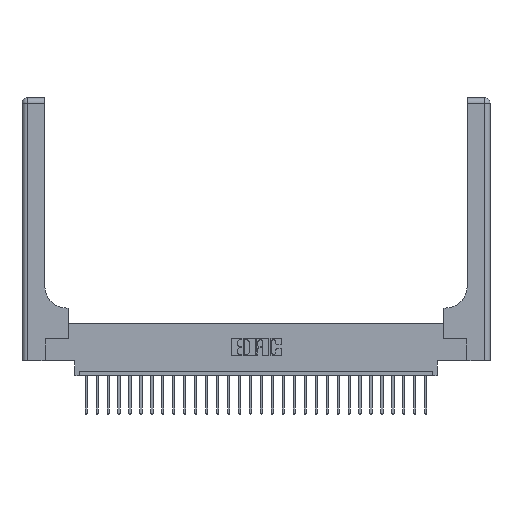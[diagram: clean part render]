
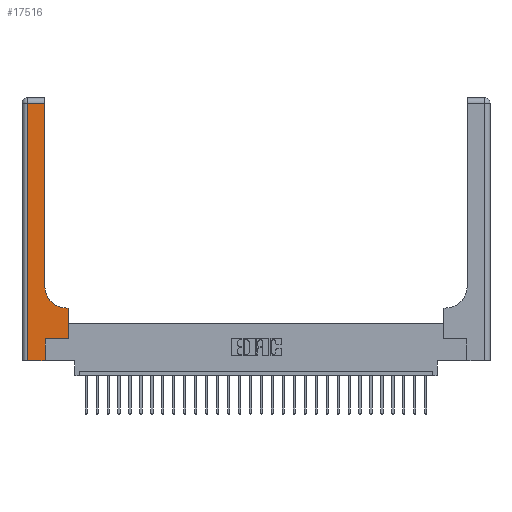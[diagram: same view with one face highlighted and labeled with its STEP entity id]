
A CAD part, top view. The second image highlights one B-rep face of the part: STEP entity #17516.
In plain terms, the highlighted planar face has unit normal (0, 0, 1).
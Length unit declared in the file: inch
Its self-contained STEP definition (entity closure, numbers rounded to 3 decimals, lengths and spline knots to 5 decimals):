
#828 = VERTEX_POINT ( 'NONE', #7912 ) ;
#926 = VECTOR ( 'NONE', #26371, 39.37008 ) ;
#1045 = LINE ( 'NONE', #6422, #16062 ) ;
#1408 = CARTESIAN_POINT ( 'NONE',  ( 0.26, 0.85, 0.37 ) ) ;
#1803 = LINE ( 'NONE', #7105, #24854 ) ;
#1862 = CARTESIAN_POINT ( 'NONE',  ( 0.51, 0.85, 0.37 ) ) ;
#2149 = ORIENTED_EDGE ( 'NONE', *, *, #23066, .T. ) ;
#2358 = LINE ( 'NONE', #22994, #5868 ) ;
#2744 = VECTOR ( 'NONE', #21874, 39.37008 ) ;
#4751 = EDGE_CURVE ( 'NONE', #7977, #6537, #1803, .T. ) ;
#5842 = CARTESIAN_POINT ( 'NONE',  ( 0.265, 0.25, 0.37 ) ) ;
#5868 = VECTOR ( 'NONE', #20844, 39.37008 ) ;
#6077 = ORIENTED_EDGE ( 'NONE', *, *, #26232, .T. ) ;
#6218 = DIRECTION ( 'NONE',  ( 0., 0., -1. ) ) ;
#6335 = DIRECTION ( 'NONE',  ( -1., 0., 0. ) ) ;
#6422 = CARTESIAN_POINT ( 'NONE',  ( 0., 2.94, 0.37 ) ) ;
#6537 = VERTEX_POINT ( 'NONE', #15780 ) ;
#6544 = CARTESIAN_POINT ( 'NONE',  ( 0.528, 0.25, 0.37 ) ) ;
#6627 = EDGE_CURVE ( 'NONE', #828, #7977, #12634, .T. ) ;
#7052 = LINE ( 'NONE', #19097, #15722 ) ;
#7105 = CARTESIAN_POINT ( 'NONE',  ( 0.265, 0., 0.37 ) ) ;
#7353 = ORIENTED_EDGE ( 'NONE', *, *, #6627, .T. ) ;
#7912 = CARTESIAN_POINT ( 'NONE',  ( 0.06, 0., 0.37 ) ) ;
#7977 = VERTEX_POINT ( 'NONE', #18852 ) ;
#7985 = EDGE_CURVE ( 'NONE', #25823, #828, #2358, .T. ) ;
#8041 = FACE_OUTER_BOUND ( 'NONE', #13156, .T. ) ;
#8305 = DIRECTION ( 'NONE',  ( 0., 0., -1. ) ) ;
#9253 = CARTESIAN_POINT ( 'NONE',  ( 0., 0., 0.37 ) ) ;
#9582 = ORIENTED_EDGE ( 'NONE', *, *, #12400, .T. ) ;
#10084 = DIRECTION ( 'NONE',  ( 1., 0., 0. ) ) ;
#11054 = DIRECTION ( 'NONE',  ( 0., 1., 0. ) ) ;
#11420 = AXIS2_PLACEMENT_3D ( 'NONE', #1862, #6218, #10084 ) ;
#11617 = ORIENTED_EDGE ( 'NONE', *, *, #22300, .T. ) ;
#12400 = EDGE_CURVE ( 'NONE', #23920, #17939, #24635, .T. ) ;
#12585 = EDGE_CURVE ( 'NONE', #6537, #16636, #26558, .T. ) ;
#12634 = LINE ( 'NONE', #9253, #2744 ) ;
#12787 = CARTESIAN_POINT ( 'NONE',  ( 0.528, 0.6, 0.37 ) ) ;
#13134 = LINE ( 'NONE', #21873, #14126 ) ;
#13156 = EDGE_LOOP ( 'NONE', ( #6077, #17796, #14498, #7353, #14496, #15392, #11617, #2149, #9582 ) ) ;
#13441 = VECTOR ( 'NONE', #13985, 39.37008 ) ;
#13769 = VERTEX_POINT ( 'NONE', #12787 ) ;
#13985 = DIRECTION ( 'NONE',  ( -1., 0., 0. ) ) ;
#14126 = VECTOR ( 'NONE', #25735, 39.37008 ) ;
#14496 = ORIENTED_EDGE ( 'NONE', *, *, #4751, .T. ) ;
#14498 = ORIENTED_EDGE ( 'NONE', *, *, #7985, .T. ) ;
#15392 = ORIENTED_EDGE ( 'NONE', *, *, #12585, .T. ) ;
#15722 = VECTOR ( 'NONE', #11054, 39.37008 ) ;
#15780 = CARTESIAN_POINT ( 'NONE',  ( 0.265, 0.25, 0.37 ) ) ;
#16014 = CARTESIAN_POINT ( 'NONE',  ( 0.51, 0.6, 0.37 ) ) ;
#16062 = VECTOR ( 'NONE', #6335, 39.37008 ) ;
#16310 = LINE ( 'NONE', #21971, #13441 ) ;
#16343 = VERTEX_POINT ( 'NONE', #21362 ) ;
#16636 = VERTEX_POINT ( 'NONE', #6544 ) ;
#17516 = ADVANCED_FACE ( 'NONE', ( #8041 ), #26511, .F. ) ;
#17796 = ORIENTED_EDGE ( 'NONE', *, *, #22095, .T. ) ;
#17939 = VERTEX_POINT ( 'NONE', #1408 ) ;
#18379 = CARTESIAN_POINT ( 'NONE',  ( 0.06, 2.94, 0.37 ) ) ;
#18852 = CARTESIAN_POINT ( 'NONE',  ( 0.265, 0., 0.37 ) ) ;
#19097 = CARTESIAN_POINT ( 'NONE',  ( 0.528, 0.25, 0.37 ) ) ;
#20844 = DIRECTION ( 'NONE',  ( 0., -1., 0. ) ) ;
#21362 = CARTESIAN_POINT ( 'NONE',  ( 0.26, 2.94, 0.37 ) ) ;
#21873 = CARTESIAN_POINT ( 'NONE',  ( 0.26, 3., 0.37 ) ) ;
#21874 = DIRECTION ( 'NONE',  ( 1., 0., 0. ) ) ;
#21971 = CARTESIAN_POINT ( 'NONE',  ( 0.26, 0.6, 0.37 ) ) ;
#22095 = EDGE_CURVE ( 'NONE', #16343, #25823, #1045, .T. ) ;
#22300 = EDGE_CURVE ( 'NONE', #16636, #13769, #7052, .T. ) ;
#22321 = AXIS2_PLACEMENT_3D ( 'NONE', #24786, #8305, #22734 ) ;
#22734 = DIRECTION ( 'NONE',  ( -1., 0., 0. ) ) ;
#22994 = CARTESIAN_POINT ( 'NONE',  ( 0.06, 3., 0.37 ) ) ;
#23066 = EDGE_CURVE ( 'NONE', #13769, #23920, #16310, .T. ) ;
#23417 = DIRECTION ( 'NONE',  ( 0., 1., 0. ) ) ;
#23920 = VERTEX_POINT ( 'NONE', #16014 ) ;
#24635 = CIRCLE ( 'NONE', #11420, 0.25 ) ;
#24786 = CARTESIAN_POINT ( 'NONE',  ( 0., 3., 0.37 ) ) ;
#24854 = VECTOR ( 'NONE', #23417, 39.37008 ) ;
#25735 = DIRECTION ( 'NONE',  ( 0., 1., 0. ) ) ;
#25823 = VERTEX_POINT ( 'NONE', #18379 ) ;
#26232 = EDGE_CURVE ( 'NONE', #17939, #16343, #13134, .T. ) ;
#26371 = DIRECTION ( 'NONE',  ( 1., 0., 0. ) ) ;
#26511 = PLANE ( 'NONE',  #22321 ) ;
#26558 = LINE ( 'NONE', #5842, #926 ) ;
